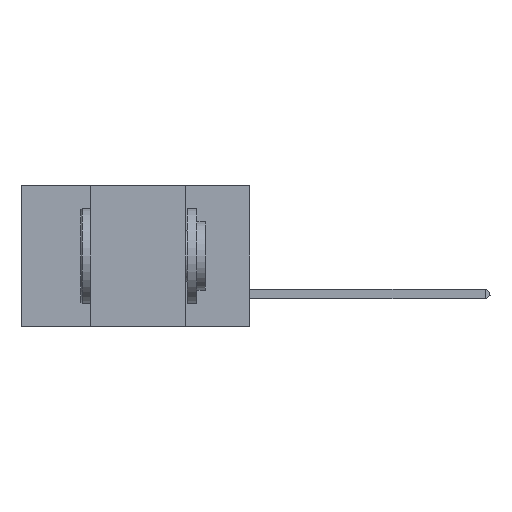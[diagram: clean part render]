
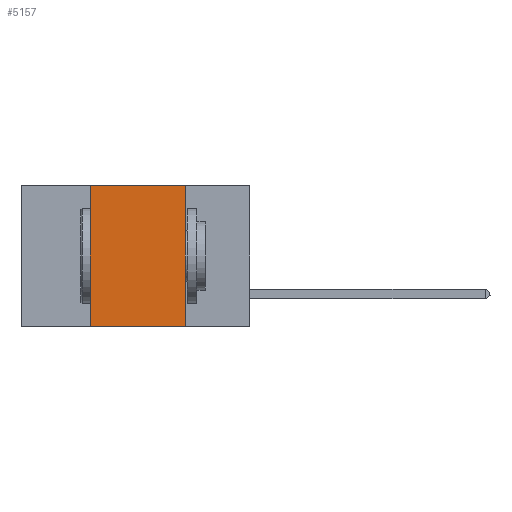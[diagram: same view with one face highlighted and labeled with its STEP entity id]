
A CAD part, left-side view. The second image highlights one B-rep face of the part: STEP entity #5157.
In plain terms, the highlighted planar face has unit normal (-1, 0, 0).
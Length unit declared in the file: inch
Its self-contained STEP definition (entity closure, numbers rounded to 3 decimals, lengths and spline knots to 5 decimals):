
#3409 = ORIENTED_EDGE ( 'NONE', *, *, #23199, .F. ) ;
#3841 = LINE ( 'NONE', #14792, #13395 ) ;
#5157 = ADVANCED_FACE ( 'NONE', ( #16088 ), #8570, .F. ) ;
#7032 = VERTEX_POINT ( 'NONE', #21156 ) ;
#7052 = CARTESIAN_POINT ( 'NONE',  ( 0., 0.17, 0. ) ) ;
#7763 = DIRECTION ( 'NONE',  ( 0., 0., 1. ) ) ;
#8570 = PLANE ( 'NONE',  #16568 ) ;
#10430 = CARTESIAN_POINT ( 'NONE',  ( 0., 0.17, 0. ) ) ;
#11601 = EDGE_CURVE ( 'NONE', #33728, #21033, #15334, .T. ) ;
#11970 = LINE ( 'NONE', #10430, #30380 ) ;
#12538 = CARTESIAN_POINT ( 'NONE',  ( 0., 0.42, 0. ) ) ;
#13395 = VECTOR ( 'NONE', #20356, 39.37008 ) ;
#14257 = DIRECTION ( 'NONE',  ( 1., 0., 0. ) ) ;
#14792 = CARTESIAN_POINT ( 'NONE',  ( 0., 0.6, -0.37 ) ) ;
#15334 = LINE ( 'NONE', #30305, #28902 ) ;
#15375 = ORIENTED_EDGE ( 'NONE', *, *, #22323, .F. ) ;
#16088 = FACE_OUTER_BOUND ( 'NONE', #26524, .T. ) ;
#16176 = DIRECTION ( 'NONE',  ( 0., 0., -1. ) ) ;
#16568 = AXIS2_PLACEMENT_3D ( 'NONE', #25406, #14257, #28077 ) ;
#17680 = VERTEX_POINT ( 'NONE', #7052 ) ;
#18418 = EDGE_CURVE ( 'NONE', #33728, #7032, #3841, .T. ) ;
#19205 = CARTESIAN_POINT ( 'NONE',  ( 0., 0.42, -0.37 ) ) ;
#20356 = DIRECTION ( 'NONE',  ( 0., -1., 0. ) ) ;
#21033 = VERTEX_POINT ( 'NONE', #12538 ) ;
#21156 = CARTESIAN_POINT ( 'NONE',  ( 0., 0.17, -0.37 ) ) ;
#22323 = EDGE_CURVE ( 'NONE', #21033, #17680, #36017, .T. ) ;
#23199 = EDGE_CURVE ( 'NONE', #17680, #7032, #11970, .T. ) ;
#25351 = CARTESIAN_POINT ( 'NONE',  ( 0., 0.6, 0. ) ) ;
#25406 = CARTESIAN_POINT ( 'NONE',  ( 0., 0.6, 0. ) ) ;
#26448 = VECTOR ( 'NONE', #31567, 39.37008 ) ;
#26524 = EDGE_LOOP ( 'NONE', ( #3409, #15375, #29769, #30067 ) ) ;
#28077 = DIRECTION ( 'NONE',  ( 0., 0., -1. ) ) ;
#28902 = VECTOR ( 'NONE', #7763, 39.37008 ) ;
#29769 = ORIENTED_EDGE ( 'NONE', *, *, #11601, .F. ) ;
#30067 = ORIENTED_EDGE ( 'NONE', *, *, #18418, .T. ) ;
#30305 = CARTESIAN_POINT ( 'NONE',  ( 0., 0.42, 0. ) ) ;
#30380 = VECTOR ( 'NONE', #16176, 39.37008 ) ;
#31567 = DIRECTION ( 'NONE',  ( 0., -1., 0. ) ) ;
#33728 = VERTEX_POINT ( 'NONE', #19205 ) ;
#36017 = LINE ( 'NONE', #25351, #26448 ) ;
